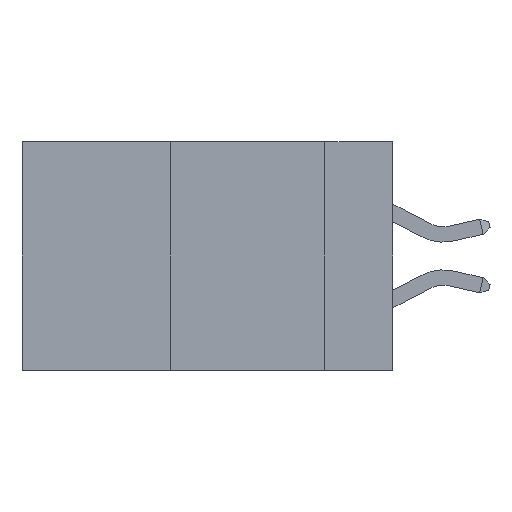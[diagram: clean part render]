
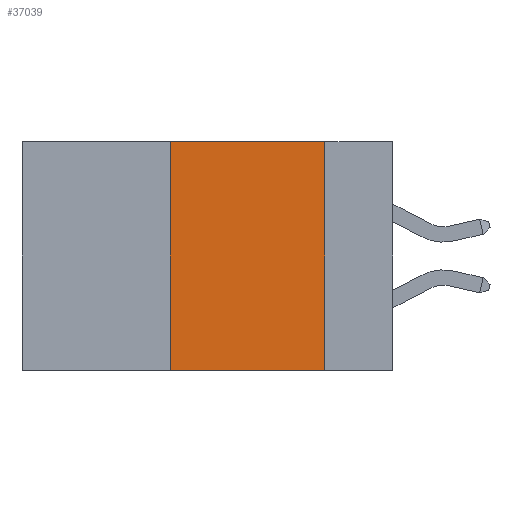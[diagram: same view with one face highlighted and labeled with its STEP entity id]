
A CAD part, left-side view. The second image highlights one B-rep face of the part: STEP entity #37039.
In plain terms, the highlighted planar face has unit normal (-1, 0, 0).
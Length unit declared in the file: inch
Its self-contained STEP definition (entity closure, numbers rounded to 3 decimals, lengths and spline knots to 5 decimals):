
#2238 = DIRECTION ( 'NONE',  ( 0., 0., 1. ) ) ;
#2401 = CARTESIAN_POINT ( 'NONE',  ( 0., 0.6, 0. ) ) ;
#2542 = VERTEX_POINT ( 'NONE', #9093 ) ;
#3994 = EDGE_CURVE ( 'NONE', #28671, #35706, #37501, .T. ) ;
#4758 = DIRECTION ( 'NONE',  ( 0., -1., 0. ) ) ;
#9093 = CARTESIAN_POINT ( 'NONE',  ( 0., 0.36, 0. ) ) ;
#10751 = VECTOR ( 'NONE', #4758, 39.37008 ) ;
#12473 = VECTOR ( 'NONE', #22791, 39.37008 ) ;
#13090 = LINE ( 'NONE', #16914, #10751 ) ;
#13699 = EDGE_CURVE ( 'NONE', #27107, #35706, #37187, .T. ) ;
#13882 = DIRECTION ( 'NONE',  ( 1., 0., 0. ) ) ;
#14486 = CARTESIAN_POINT ( 'NONE',  ( 0., 0.36, -0.37 ) ) ;
#16092 = CARTESIAN_POINT ( 'NONE',  ( 0., 0.11, 0. ) ) ;
#16914 = CARTESIAN_POINT ( 'NONE',  ( 0., 0.6, 0. ) ) ;
#17017 = DIRECTION ( 'NONE',  ( 0., 0., -1. ) ) ;
#18083 = VECTOR ( 'NONE', #2238, 39.37008 ) ;
#19642 = EDGE_LOOP ( 'NONE', ( #37028, #20305, #25838, #24788 ) ) ;
#20305 = ORIENTED_EDGE ( 'NONE', *, *, #34792, .F. ) ;
#22236 = EDGE_CURVE ( 'NONE', #27107, #2542, #26017, .T. ) ;
#22314 = DIRECTION ( 'NONE',  ( 0., 0., -1. ) ) ;
#22791 = DIRECTION ( 'NONE',  ( 0., -1., 0. ) ) ;
#23245 = CARTESIAN_POINT ( 'NONE',  ( 0., 0.11, -0.37 ) ) ;
#24788 = ORIENTED_EDGE ( 'NONE', *, *, #13699, .T. ) ;
#25838 = ORIENTED_EDGE ( 'NONE', *, *, #22236, .F. ) ;
#26017 = LINE ( 'NONE', #37542, #18083 ) ;
#27107 = VERTEX_POINT ( 'NONE', #14486 ) ;
#28671 = VERTEX_POINT ( 'NONE', #16092 ) ;
#28910 = PLANE ( 'NONE',  #33160 ) ;
#31311 = CARTESIAN_POINT ( 'NONE',  ( 0., 0.11, 0. ) ) ;
#32847 = VECTOR ( 'NONE', #22314, 39.37008 ) ;
#33160 = AXIS2_PLACEMENT_3D ( 'NONE', #2401, #13882, #17017 ) ;
#34172 = FACE_OUTER_BOUND ( 'NONE', #19642, .T. ) ;
#34775 = CARTESIAN_POINT ( 'NONE',  ( 0., 0.6, -0.37 ) ) ;
#34792 = EDGE_CURVE ( 'NONE', #2542, #28671, #13090, .T. ) ;
#35706 = VERTEX_POINT ( 'NONE', #23245 ) ;
#37028 = ORIENTED_EDGE ( 'NONE', *, *, #3994, .F. ) ;
#37039 = ADVANCED_FACE ( 'NONE', ( #34172 ), #28910, .F. ) ;
#37187 = LINE ( 'NONE', #34775, #12473 ) ;
#37501 = LINE ( 'NONE', #31311, #32847 ) ;
#37542 = CARTESIAN_POINT ( 'NONE',  ( 0., 0.36, 0. ) ) ;
